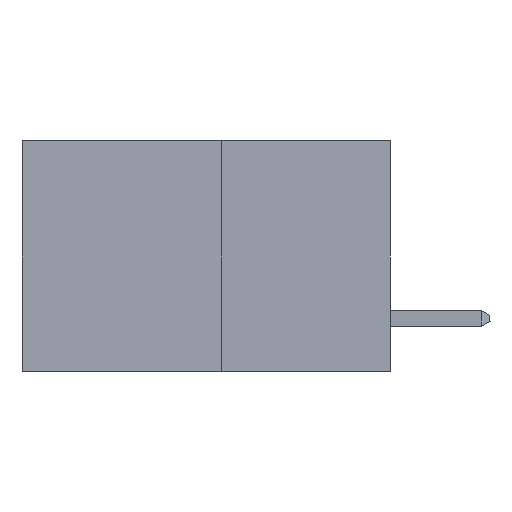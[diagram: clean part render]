
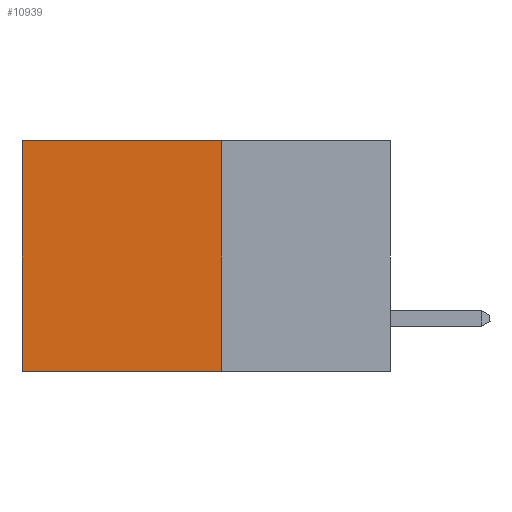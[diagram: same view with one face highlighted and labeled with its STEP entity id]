
A CAD part, left-side view. The second image highlights one B-rep face of the part: STEP entity #10939.
In plain terms, the highlighted planar face has unit normal (-1, 0, 0).
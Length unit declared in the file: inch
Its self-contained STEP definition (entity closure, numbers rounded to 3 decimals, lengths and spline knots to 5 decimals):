
#1370 = ORIENTED_EDGE ( 'NONE', *, *, #6020, .F. ) ;
#4139 = VECTOR ( 'NONE', #12927, 39.37008 ) ;
#5070 = EDGE_LOOP ( 'NONE', ( #23391, #13315, #1370, #10890 ) ) ;
#6020 = EDGE_CURVE ( 'NONE', #11733, #10201, #19308, .T. ) ;
#6206 = AXIS2_PLACEMENT_3D ( 'NONE', #14587, #11100, #12829 ) ;
#8091 = VERTEX_POINT ( 'NONE', #17642 ) ;
#8153 = DIRECTION ( 'NONE',  ( 0., 1., 0. ) ) ;
#9088 = CARTESIAN_POINT ( 'NONE',  ( 0.277, 0.59, -0.37 ) ) ;
#10201 = VERTEX_POINT ( 'NONE', #15803 ) ;
#10593 = LINE ( 'NONE', #16977, #19778 ) ;
#10890 = ORIENTED_EDGE ( 'NONE', *, *, #18101, .T. ) ;
#10939 = ADVANCED_FACE ( 'NONE', ( #15166 ), #10983, .F. ) ;
#10983 = PLANE ( 'NONE',  #6206 ) ;
#11100 = DIRECTION ( 'NONE',  ( 1., 0., 0. ) ) ;
#11196 = CARTESIAN_POINT ( 'NONE',  ( 0.277, 0.27, 0. ) ) ;
#11733 = VERTEX_POINT ( 'NONE', #11196 ) ;
#12829 = DIRECTION ( 'NONE',  ( 0., 0., -1. ) ) ;
#12927 = DIRECTION ( 'NONE',  ( 0., 0., -1. ) ) ;
#12970 = DIRECTION ( 'NONE',  ( 0., 0., -1. ) ) ;
#13315 = ORIENTED_EDGE ( 'NONE', *, *, #15437, .F. ) ;
#13570 = VECTOR ( 'NONE', #12970, 39.37008 ) ;
#14139 = LINE ( 'NONE', #22126, #13570 ) ;
#14587 = CARTESIAN_POINT ( 'NONE',  ( 0.277, 0.27, -0.37 ) ) ;
#15166 = FACE_OUTER_BOUND ( 'NONE', #5070, .T. ) ;
#15437 = EDGE_CURVE ( 'NONE', #10201, #20948, #10593, .T. ) ;
#15803 = CARTESIAN_POINT ( 'NONE',  ( 0.277, 0.27, -0.37 ) ) ;
#16249 = LINE ( 'NONE', #17250, #18861 ) ;
#16977 = CARTESIAN_POINT ( 'NONE',  ( 0.277, 0.27, -0.37 ) ) ;
#17250 = CARTESIAN_POINT ( 'NONE',  ( 0.277, 0.27, 0. ) ) ;
#17642 = CARTESIAN_POINT ( 'NONE',  ( 0.277, 0.59, 0. ) ) ;
#18101 = EDGE_CURVE ( 'NONE', #11733, #8091, #16249, .T. ) ;
#18844 = DIRECTION ( 'NONE',  ( 0., 1., 0. ) ) ;
#18861 = VECTOR ( 'NONE', #8153, 39.37008 ) ;
#19308 = LINE ( 'NONE', #22079, #4139 ) ;
#19778 = VECTOR ( 'NONE', #18844, 39.37008 ) ;
#20948 = VERTEX_POINT ( 'NONE', #9088 ) ;
#21022 = EDGE_CURVE ( 'NONE', #8091, #20948, #14139, .T. ) ;
#22079 = CARTESIAN_POINT ( 'NONE',  ( 0.277, 0.27, -0.37 ) ) ;
#22126 = CARTESIAN_POINT ( 'NONE',  ( 0.277, 0.59, -0.37 ) ) ;
#23391 = ORIENTED_EDGE ( 'NONE', *, *, #21022, .T. ) ;
